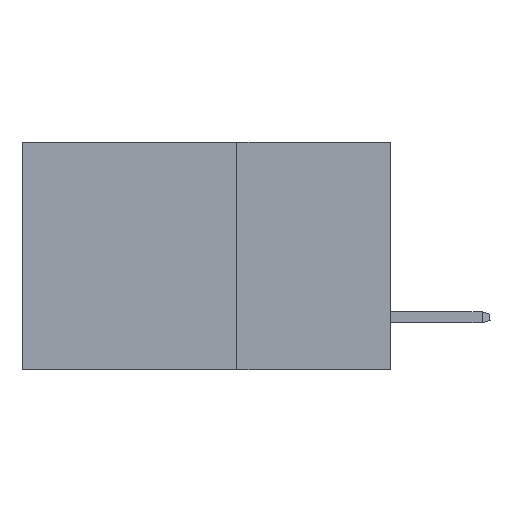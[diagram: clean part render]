
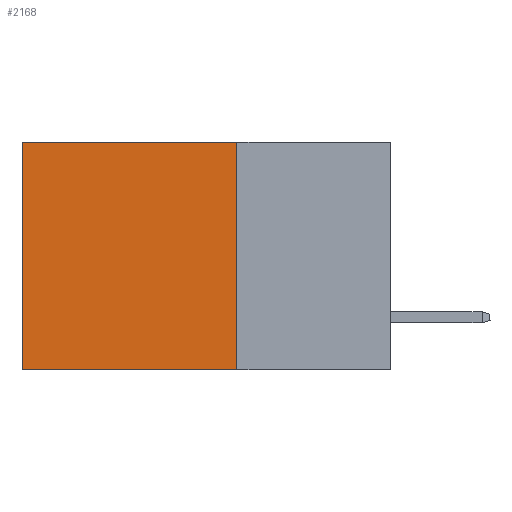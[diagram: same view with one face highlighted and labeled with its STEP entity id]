
A CAD part, left-side view. The second image highlights one B-rep face of the part: STEP entity #2168.
In plain terms, the highlighted planar face has unit normal (-1, 0, 0).
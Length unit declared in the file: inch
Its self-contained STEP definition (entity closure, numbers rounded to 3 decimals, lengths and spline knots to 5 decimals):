
#392 = VERTEX_POINT ( 'NONE', #9655 ) ;
#887 = EDGE_CURVE ( 'NONE', #10755, #9125, #9001, .T. ) ;
#1249 = LINE ( 'NONE', #13693, #7100 ) ;
#1400 = EDGE_LOOP ( 'NONE', ( #16136, #6472, #7160, #10428 ) ) ;
#1887 = CARTESIAN_POINT ( 'NONE',  ( 0.2875, 0.25, 0. ) ) ;
#1902 = DIRECTION ( 'NONE',  ( 0., 1., 0. ) ) ;
#2168 = ADVANCED_FACE ( 'NONE', ( #9391 ), #14802, .F. ) ;
#2408 = EDGE_CURVE ( 'NONE', #16803, #392, #1249, .T. ) ;
#3245 = DIRECTION ( 'NONE',  ( 0., 1., 0. ) ) ;
#3695 = CARTESIAN_POINT ( 'NONE',  ( 0.2875, 0.6, 0. ) ) ;
#4108 = VECTOR ( 'NONE', #9148, 39.37008 ) ;
#4633 = CARTESIAN_POINT ( 'NONE',  ( 0.2875, 0.25, 0. ) ) ;
#6381 = DIRECTION ( 'NONE',  ( 0., 0., -1. ) ) ;
#6472 = ORIENTED_EDGE ( 'NONE', *, *, #887, .F. ) ;
#6550 = VECTOR ( 'NONE', #1902, 39.37008 ) ;
#6942 = LINE ( 'NONE', #1887, #13087 ) ;
#7024 = DIRECTION ( 'NONE',  ( 0., 0., -1. ) ) ;
#7100 = VECTOR ( 'NONE', #3245, 39.37008 ) ;
#7160 = ORIENTED_EDGE ( 'NONE', *, *, #13329, .F. ) ;
#8267 = CARTESIAN_POINT ( 'NONE',  ( 0.2875, 0.25, 0. ) ) ;
#8653 = CARTESIAN_POINT ( 'NONE',  ( 0.2875, 0.25, -0.37 ) ) ;
#8658 = AXIS2_PLACEMENT_3D ( 'NONE', #4633, #14278, #6381 ) ;
#9001 = LINE ( 'NONE', #9690, #6550 ) ;
#9123 = EDGE_CURVE ( 'NONE', #392, #9125, #13722, .T. ) ;
#9125 = VERTEX_POINT ( 'NONE', #10351 ) ;
#9148 = DIRECTION ( 'NONE',  ( 0., 0., -1. ) ) ;
#9391 = FACE_OUTER_BOUND ( 'NONE', #1400, .T. ) ;
#9655 = CARTESIAN_POINT ( 'NONE',  ( 0.2875, 0.6, 0. ) ) ;
#9690 = CARTESIAN_POINT ( 'NONE',  ( 0.2875, 0.25, -0.37 ) ) ;
#10351 = CARTESIAN_POINT ( 'NONE',  ( 0.2875, 0.6, -0.37 ) ) ;
#10428 = ORIENTED_EDGE ( 'NONE', *, *, #2408, .T. ) ;
#10755 = VERTEX_POINT ( 'NONE', #8653 ) ;
#13087 = VECTOR ( 'NONE', #7024, 39.37008 ) ;
#13329 = EDGE_CURVE ( 'NONE', #16803, #10755, #6942, .T. ) ;
#13693 = CARTESIAN_POINT ( 'NONE',  ( 0.2875, 0.25, 0. ) ) ;
#13722 = LINE ( 'NONE', #3695, #4108 ) ;
#14278 = DIRECTION ( 'NONE',  ( 1., 0., 0. ) ) ;
#14802 = PLANE ( 'NONE',  #8658 ) ;
#16136 = ORIENTED_EDGE ( 'NONE', *, *, #9123, .T. ) ;
#16803 = VERTEX_POINT ( 'NONE', #8267 ) ;
